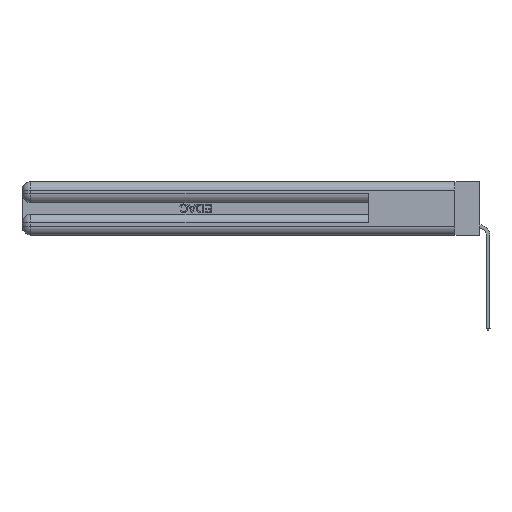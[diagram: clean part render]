
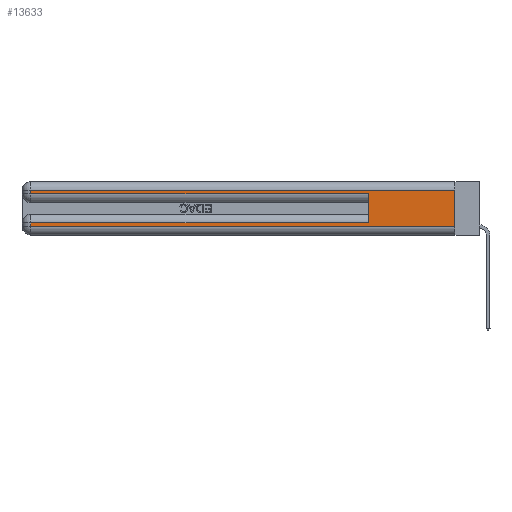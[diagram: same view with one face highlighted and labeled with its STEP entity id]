
A CAD part, left-side view. The second image highlights one B-rep face of the part: STEP entity #13633.
In plain terms, the highlighted planar face has unit normal (-1, 0, 0).
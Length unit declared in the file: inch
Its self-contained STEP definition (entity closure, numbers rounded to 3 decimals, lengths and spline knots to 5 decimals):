
#870 = VERTEX_POINT ( 'NONE', #13991 ) ;
#2228 = EDGE_LOOP ( 'NONE', ( #4607, #8623, #13499, #2250, #34285, #15879, #6332, #2508 ) ) ;
#2250 = ORIENTED_EDGE ( 'NONE', *, *, #23817, .T. ) ;
#2508 = ORIENTED_EDGE ( 'NONE', *, *, #10354, .T. ) ;
#2535 = EDGE_CURVE ( 'NONE', #14454, #3892, #22916, .T. ) ;
#3406 = CARTESIAN_POINT ( 'NONE',  ( 0., 2.94, 0.37 ) ) ;
#3750 = CARTESIAN_POINT ( 'NONE',  ( 0., 2.94, 0.085 ) ) ;
#3892 = VERTEX_POINT ( 'NONE', #14541 ) ;
#4192 = VECTOR ( 'NONE', #28923, 39.37008 ) ;
#4341 = CARTESIAN_POINT ( 'NONE',  ( 0., 0., 0.37 ) ) ;
#4492 = CARTESIAN_POINT ( 'NONE',  ( 0., 0., 0.31 ) ) ;
#4493 = VERTEX_POINT ( 'NONE', #25073 ) ;
#4607 = ORIENTED_EDGE ( 'NONE', *, *, #8135, .F. ) ;
#5442 = LINE ( 'NONE', #4492, #12627 ) ;
#6332 = ORIENTED_EDGE ( 'NONE', *, *, #2535, .T. ) ;
#7156 = VECTOR ( 'NONE', #9590, 39.37008 ) ;
#7231 = CARTESIAN_POINT ( 'NONE',  ( 0., 2.94, 0.37 ) ) ;
#7240 = CARTESIAN_POINT ( 'NONE',  ( 0., 0., 0.31 ) ) ;
#8135 = EDGE_CURVE ( 'NONE', #13026, #14130, #27566, .T. ) ;
#8363 = CARTESIAN_POINT ( 'NONE',  ( 0., 0.6, 0.285 ) ) ;
#8623 = ORIENTED_EDGE ( 'NONE', *, *, #23905, .T. ) ;
#9094 = AXIS2_PLACEMENT_3D ( 'NONE', #4341, #33952, #17892 ) ;
#9590 = DIRECTION ( 'NONE',  ( 0., -1., 0. ) ) ;
#9632 = CARTESIAN_POINT ( 'NONE',  ( 0., 0.6, 0.145 ) ) ;
#10018 = VECTOR ( 'NONE', #15339, 39.37008 ) ;
#10185 = CARTESIAN_POINT ( 'NONE',  ( 0., 0., 0.085 ) ) ;
#10311 = VERTEX_POINT ( 'NONE', #16525 ) ;
#10354 = EDGE_CURVE ( 'NONE', #3892, #14130, #29777, .T. ) ;
#10738 = FACE_OUTER_BOUND ( 'NONE', #2228, .T. ) ;
#11189 = EDGE_CURVE ( 'NONE', #870, #4493, #23453, .T. ) ;
#12326 = DIRECTION ( 'NONE',  ( 0., 0., 1. ) ) ;
#12622 = LINE ( 'NONE', #9632, #26058 ) ;
#12627 = VECTOR ( 'NONE', #20645, 39.37008 ) ;
#13026 = VERTEX_POINT ( 'NONE', #7240 ) ;
#13499 = ORIENTED_EDGE ( 'NONE', *, *, #11189, .T. ) ;
#13633 = ADVANCED_FACE ( 'NONE', ( #10738 ), #31229, .F. ) ;
#13991 = CARTESIAN_POINT ( 'NONE',  ( 0., 2.94, 0.31 ) ) ;
#14130 = VERTEX_POINT ( 'NONE', #31278 ) ;
#14307 = LINE ( 'NONE', #22985, #7156 ) ;
#14454 = VERTEX_POINT ( 'NONE', #3750 ) ;
#14541 = CARTESIAN_POINT ( 'NONE',  ( 0., 2.94, 0.06 ) ) ;
#15339 = DIRECTION ( 'NONE',  ( 0., 0., -1. ) ) ;
#15879 = ORIENTED_EDGE ( 'NONE', *, *, #20121, .T. ) ;
#16335 = VERTEX_POINT ( 'NONE', #8363 ) ;
#16379 = VECTOR ( 'NONE', #32702, 39.37008 ) ;
#16525 = CARTESIAN_POINT ( 'NONE',  ( 0., 0.6, 0.085 ) ) ;
#16644 = CARTESIAN_POINT ( 'NONE',  ( 0., 0., 0.06 ) ) ;
#16852 = LINE ( 'NONE', #10185, #4192 ) ;
#17892 = DIRECTION ( 'NONE',  ( 0., 0., -1. ) ) ;
#20121 = EDGE_CURVE ( 'NONE', #10311, #14454, #16852, .T. ) ;
#20645 = DIRECTION ( 'NONE',  ( 0., 1., 0. ) ) ;
#22916 = LINE ( 'NONE', #3406, #23733 ) ;
#22985 = CARTESIAN_POINT ( 'NONE',  ( 0., 0., 0.285 ) ) ;
#23221 = EDGE_CURVE ( 'NONE', #10311, #16335, #12622, .T. ) ;
#23453 = LINE ( 'NONE', #7231, #10018 ) ;
#23733 = VECTOR ( 'NONE', #27635, 39.37008 ) ;
#23817 = EDGE_CURVE ( 'NONE', #4493, #16335, #14307, .T. ) ;
#23905 = EDGE_CURVE ( 'NONE', #13026, #870, #5442, .T. ) ;
#25073 = CARTESIAN_POINT ( 'NONE',  ( 0., 2.94, 0.285 ) ) ;
#26058 = VECTOR ( 'NONE', #12326, 39.37008 ) ;
#27566 = LINE ( 'NONE', #30950, #34683 ) ;
#27635 = DIRECTION ( 'NONE',  ( 0., 0., -1. ) ) ;
#28923 = DIRECTION ( 'NONE',  ( 0., 1., 0. ) ) ;
#29777 = LINE ( 'NONE', #16644, #16379 ) ;
#30950 = CARTESIAN_POINT ( 'NONE',  ( 0., 0., 0.37 ) ) ;
#31066 = DIRECTION ( 'NONE',  ( 0., 0., -1. ) ) ;
#31229 = PLANE ( 'NONE',  #9094 ) ;
#31278 = CARTESIAN_POINT ( 'NONE',  ( 0., 0., 0.06 ) ) ;
#32702 = DIRECTION ( 'NONE',  ( 0., -1., 0. ) ) ;
#33952 = DIRECTION ( 'NONE',  ( 1., 0., 0. ) ) ;
#34285 = ORIENTED_EDGE ( 'NONE', *, *, #23221, .F. ) ;
#34683 = VECTOR ( 'NONE', #31066, 39.37008 ) ;
